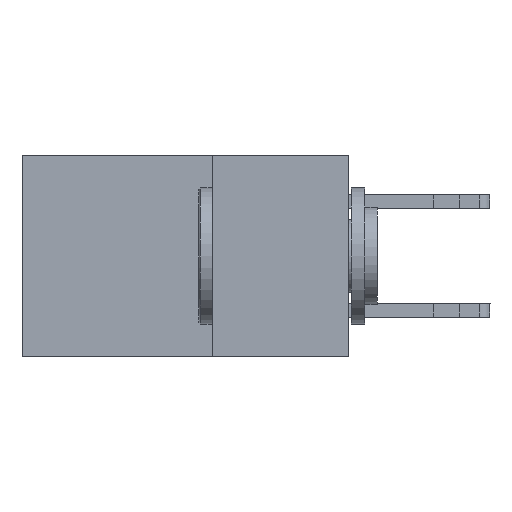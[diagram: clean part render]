
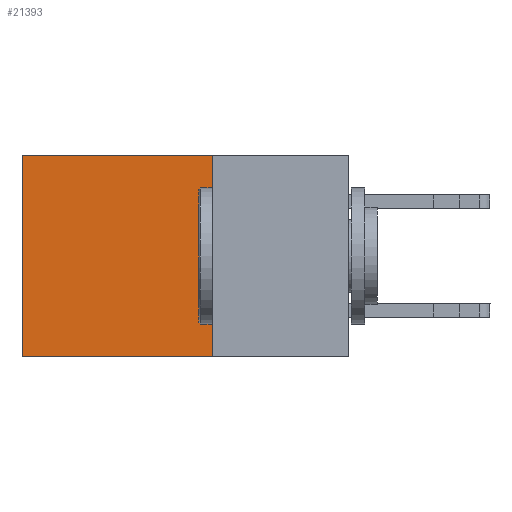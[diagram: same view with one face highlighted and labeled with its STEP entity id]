
A CAD part, left-side view. The second image highlights one B-rep face of the part: STEP entity #21393.
In plain terms, the highlighted planar face has unit normal (-1, 0, 0).
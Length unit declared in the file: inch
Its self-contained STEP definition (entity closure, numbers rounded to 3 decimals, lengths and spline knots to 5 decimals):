
#58 = CARTESIAN_POINT ( 'NONE',  ( 0.2615, 0.25, -0.37 ) ) ;
#351 = EDGE_LOOP ( 'NONE', ( #20175, #17586, #19000, #5319 ) ) ;
#1816 = DIRECTION ( 'NONE',  ( 0., 0., -1. ) ) ;
#3169 = CARTESIAN_POINT ( 'NONE',  ( 0.2615, 0.25, -0.37 ) ) ;
#3329 = VERTEX_POINT ( 'NONE', #3169 ) ;
#4560 = VECTOR ( 'NONE', #21144, 39.37008 ) ;
#5085 = LINE ( 'NONE', #9637, #4560 ) ;
#5319 = ORIENTED_EDGE ( 'NONE', *, *, #10954, .T. ) ;
#6215 = LINE ( 'NONE', #8860, #6750 ) ;
#6655 = CARTESIAN_POINT ( 'NONE',  ( 0.2615, 0.25, 0. ) ) ;
#6750 = VECTOR ( 'NONE', #20356, 39.37008 ) ;
#7026 = EDGE_CURVE ( 'NONE', #19523, #13089, #6215, .T. ) ;
#7087 = AXIS2_PLACEMENT_3D ( 'NONE', #58, #11688, #1816 ) ;
#7681 = CARTESIAN_POINT ( 'NONE',  ( 0.2615, 0.6, -0.37 ) ) ;
#8436 = PLANE ( 'NONE',  #7087 ) ;
#8776 = CARTESIAN_POINT ( 'NONE',  ( 0.2615, 0.6, 0. ) ) ;
#8860 = CARTESIAN_POINT ( 'NONE',  ( 0.2615, 0.6, -0.37 ) ) ;
#9637 = CARTESIAN_POINT ( 'NONE',  ( 0.2615, 0.25, -0.37 ) ) ;
#10258 = LINE ( 'NONE', #6655, #13583 ) ;
#10295 = DIRECTION ( 'NONE',  ( 0., 1., 0. ) ) ;
#10954 = EDGE_CURVE ( 'NONE', #19947, #19523, #10258, .T. ) ;
#11292 = CARTESIAN_POINT ( 'NONE',  ( 0.2615, 0.25, 0. ) ) ;
#11688 = DIRECTION ( 'NONE',  ( 1., 0., 0. ) ) ;
#11865 = CARTESIAN_POINT ( 'NONE',  ( 0.2615, 0.25, -0.37 ) ) ;
#13021 = EDGE_CURVE ( 'NONE', #3329, #13089, #13761, .T. ) ;
#13089 = VERTEX_POINT ( 'NONE', #7681 ) ;
#13583 = VECTOR ( 'NONE', #14835, 39.37008 ) ;
#13761 = LINE ( 'NONE', #11865, #17665 ) ;
#14835 = DIRECTION ( 'NONE',  ( 0., 1., 0. ) ) ;
#15093 = FACE_OUTER_BOUND ( 'NONE', #351, .T. ) ;
#17586 = ORIENTED_EDGE ( 'NONE', *, *, #13021, .F. ) ;
#17665 = VECTOR ( 'NONE', #10295, 39.37008 ) ;
#19000 = ORIENTED_EDGE ( 'NONE', *, *, #21236, .F. ) ;
#19523 = VERTEX_POINT ( 'NONE', #8776 ) ;
#19947 = VERTEX_POINT ( 'NONE', #11292 ) ;
#20175 = ORIENTED_EDGE ( 'NONE', *, *, #7026, .T. ) ;
#20356 = DIRECTION ( 'NONE',  ( 0., 0., -1. ) ) ;
#21144 = DIRECTION ( 'NONE',  ( 0., 0., -1. ) ) ;
#21236 = EDGE_CURVE ( 'NONE', #19947, #3329, #5085, .T. ) ;
#21393 = ADVANCED_FACE ( 'NONE', ( #15093 ), #8436, .F. ) ;
